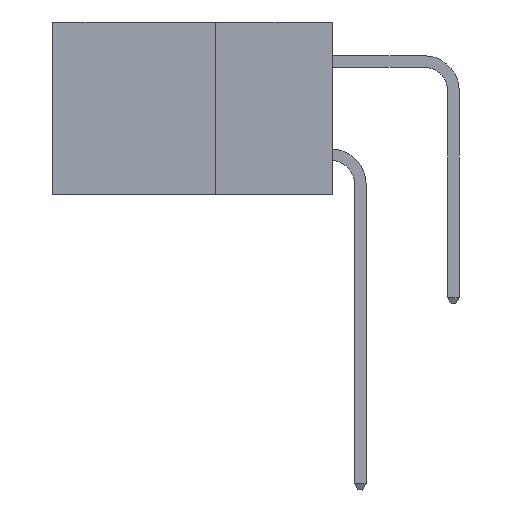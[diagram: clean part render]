
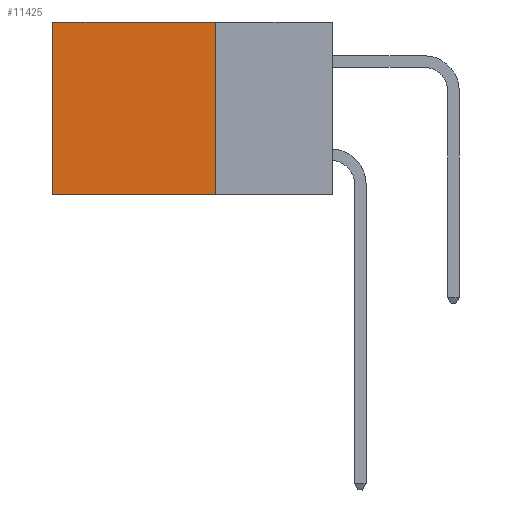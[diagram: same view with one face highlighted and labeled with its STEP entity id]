
A CAD part, left-side view. The second image highlights one B-rep face of the part: STEP entity #11425.
In plain terms, the highlighted planar face has unit normal (-1, 0, 0).
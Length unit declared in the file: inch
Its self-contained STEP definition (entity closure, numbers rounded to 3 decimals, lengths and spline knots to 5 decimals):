
#347 = VECTOR ( 'NONE', #9398, 39.37008 ) ;
#2318 = AXIS2_PLACEMENT_3D ( 'NONE', #3660, #8941, #2947 ) ;
#2540 = EDGE_CURVE ( 'NONE', #4630, #5538, #7091, .T. ) ;
#2947 = DIRECTION ( 'NONE',  ( 0., 0., -1. ) ) ;
#3626 = VECTOR ( 'NONE', #4638, 39.37008 ) ;
#3660 = CARTESIAN_POINT ( 'NONE',  ( 0.298, 0.25, 0. ) ) ;
#4277 = VERTEX_POINT ( 'NONE', #11325 ) ;
#4630 = VERTEX_POINT ( 'NONE', #8425 ) ;
#4638 = DIRECTION ( 'NONE',  ( 0., 0., -1. ) ) ;
#5003 = ORIENTED_EDGE ( 'NONE', *, *, #5468, .T. ) ;
#5207 = LINE ( 'NONE', #9840, #11706 ) ;
#5468 = EDGE_CURVE ( 'NONE', #4277, #9579, #11797, .T. ) ;
#5538 = VERTEX_POINT ( 'NONE', #13612 ) ;
#6351 = CARTESIAN_POINT ( 'NONE',  ( 0.298, 0.6, 0. ) ) ;
#6980 = LINE ( 'NONE', #8173, #347 ) ;
#7091 = LINE ( 'NONE', #13588, #3626 ) ;
#8173 = CARTESIAN_POINT ( 'NONE',  ( 0.298, 0.25, -0.37 ) ) ;
#8425 = CARTESIAN_POINT ( 'NONE',  ( 0.298, 0.25, 0. ) ) ;
#8483 = ORIENTED_EDGE ( 'NONE', *, *, #15452, .F. ) ;
#8733 = EDGE_CURVE ( 'NONE', #4630, #4277, #5207, .T. ) ;
#8767 = VECTOR ( 'NONE', #12118, 39.37008 ) ;
#8941 = DIRECTION ( 'NONE',  ( 1., 0., 0. ) ) ;
#8978 = PLANE ( 'NONE',  #2318 ) ;
#9398 = DIRECTION ( 'NONE',  ( 0., 1., 0. ) ) ;
#9579 = VERTEX_POINT ( 'NONE', #9716 ) ;
#9716 = CARTESIAN_POINT ( 'NONE',  ( 0.298, 0.6, -0.37 ) ) ;
#9780 = DIRECTION ( 'NONE',  ( 0., 1., 0. ) ) ;
#9840 = CARTESIAN_POINT ( 'NONE',  ( 0.298, 0.25, 0. ) ) ;
#10206 = EDGE_LOOP ( 'NONE', ( #5003, #8483, #11909, #15322 ) ) ;
#11325 = CARTESIAN_POINT ( 'NONE',  ( 0.298, 0.6, 0. ) ) ;
#11425 = ADVANCED_FACE ( 'NONE', ( #11556 ), #8978, .F. ) ;
#11556 = FACE_OUTER_BOUND ( 'NONE', #10206, .T. ) ;
#11706 = VECTOR ( 'NONE', #9780, 39.37008 ) ;
#11797 = LINE ( 'NONE', #6351, #8767 ) ;
#11909 = ORIENTED_EDGE ( 'NONE', *, *, #2540, .F. ) ;
#12118 = DIRECTION ( 'NONE',  ( 0., 0., -1. ) ) ;
#13588 = CARTESIAN_POINT ( 'NONE',  ( 0.298, 0.25, 0. ) ) ;
#13612 = CARTESIAN_POINT ( 'NONE',  ( 0.298, 0.25, -0.37 ) ) ;
#15322 = ORIENTED_EDGE ( 'NONE', *, *, #8733, .T. ) ;
#15452 = EDGE_CURVE ( 'NONE', #5538, #9579, #6980, .T. ) ;
